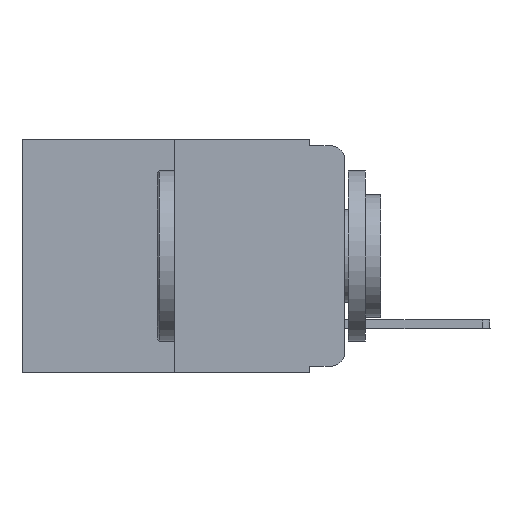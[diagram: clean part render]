
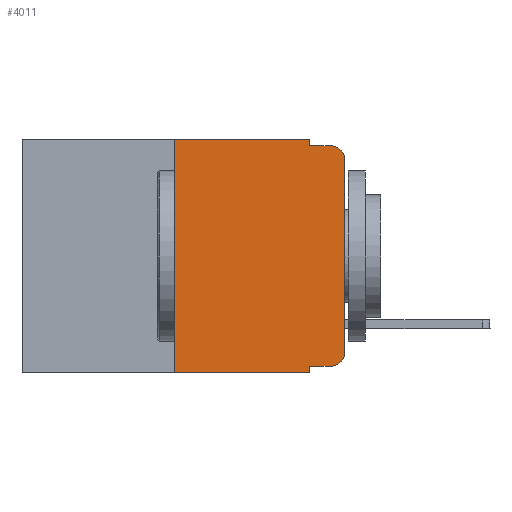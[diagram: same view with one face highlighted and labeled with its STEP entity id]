
A CAD part, left-side view. The second image highlights one B-rep face of the part: STEP entity #4011.
In plain terms, the highlighted planar face has unit normal (-1, 0, 0).
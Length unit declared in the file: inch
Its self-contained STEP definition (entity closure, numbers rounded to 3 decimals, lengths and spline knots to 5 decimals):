
#27 = VECTOR ( 'NONE', #8465, 39.37008 ) ;
#137 = CARTESIAN_POINT ( 'NONE',  ( 0., 0.25, 0. ) ) ;
#147 = DIRECTION ( 'NONE',  ( 0., -1., 0. ) ) ;
#211 = VECTOR ( 'NONE', #1115, 39.37008 ) ;
#227 = CARTESIAN_POINT ( 'NONE',  ( 0., 0.051, -0.01 ) ) ;
#622 = VERTEX_POINT ( 'NONE', #4128 ) ;
#785 = EDGE_CURVE ( 'NONE', #6028, #1741, #1272, .T. ) ;
#848 = VERTEX_POINT ( 'NONE', #7690 ) ;
#938 = CARTESIAN_POINT ( 'NONE',  ( 0., 0.473, 0. ) ) ;
#985 = CIRCLE ( 'NONE', #3263, 0.02 ) ;
#1009 = VECTOR ( 'NONE', #7620, 39.37008 ) ;
#1115 = DIRECTION ( 'NONE',  ( 0., 0., -1. ) ) ;
#1272 = LINE ( 'NONE', #227, #1009 ) ;
#1364 = CIRCLE ( 'NONE', #2346, 0.02 ) ;
#1446 = CARTESIAN_POINT ( 'NONE',  ( 0., 0.25, -0.343 ) ) ;
#1741 = VERTEX_POINT ( 'NONE', #6923 ) ;
#1876 = EDGE_CURVE ( 'NONE', #622, #10513, #1364, .T. ) ;
#1916 = CARTESIAN_POINT ( 'NONE',  ( 0., 0.473, 0. ) ) ;
#1956 = LINE ( 'NONE', #5800, #9907 ) ;
#2013 = LINE ( 'NONE', #9320, #211 ) ;
#2055 = VERTEX_POINT ( 'NONE', #137 ) ;
#2346 = AXIS2_PLACEMENT_3D ( 'NONE', #5459, #7097, #10304 ) ;
#2464 = CARTESIAN_POINT ( 'NONE',  ( 0., 0.02, -0.03 ) ) ;
#2688 = ORIENTED_EDGE ( 'NONE', *, *, #8754, .F. ) ;
#2755 = LINE ( 'NONE', #10289, #8506 ) ;
#2963 = DIRECTION ( 'NONE',  ( 0., 0., -1. ) ) ;
#3263 = AXIS2_PLACEMENT_3D ( 'NONE', #2464, #9793, #2963 ) ;
#3369 = CARTESIAN_POINT ( 'NONE',  ( 0., 0.051, 0. ) ) ;
#3418 = CARTESIAN_POINT ( 'NONE',  ( 0., 0., -0.03 ) ) ;
#3681 = DIRECTION ( 'NONE',  ( 0., 0., 1. ) ) ;
#3686 = EDGE_CURVE ( 'NONE', #10513, #10509, #2755, .T. ) ;
#4011 = ADVANCED_FACE ( 'NONE', ( #4802 ), #9938, .F. ) ;
#4128 = CARTESIAN_POINT ( 'NONE',  ( 0., 0.02, -0.333 ) ) ;
#4333 = ORIENTED_EDGE ( 'NONE', *, *, #5202, .T. ) ;
#4451 = VERTEX_POINT ( 'NONE', #1446 ) ;
#4654 = EDGE_CURVE ( 'NONE', #10509, #1741, #985, .T. ) ;
#4802 = FACE_OUTER_BOUND ( 'NONE', #8972, .T. ) ;
#5042 = EDGE_CURVE ( 'NONE', #6371, #848, #2013, .T. ) ;
#5116 = ORIENTED_EDGE ( 'NONE', *, *, #1876, .T. ) ;
#5119 = DIRECTION ( 'NONE',  ( 0., 0., -1. ) ) ;
#5202 = EDGE_CURVE ( 'NONE', #4451, #848, #7410, .T. ) ;
#5224 = VECTOR ( 'NONE', #7140, 39.37008 ) ;
#5459 = CARTESIAN_POINT ( 'NONE',  ( 0., 0.02, -0.313 ) ) ;
#5463 = CARTESIAN_POINT ( 'NONE',  ( 0., 0.473, -0.343 ) ) ;
#5565 = LINE ( 'NONE', #1916, #27 ) ;
#5712 = LINE ( 'NONE', #3369, #10300 ) ;
#5800 = CARTESIAN_POINT ( 'NONE',  ( 0., 0.051, -0.333 ) ) ;
#5867 = DIRECTION ( 'NONE',  ( 0., 0., -1. ) ) ;
#6028 = VERTEX_POINT ( 'NONE', #9392 ) ;
#6371 = VERTEX_POINT ( 'NONE', #9233 ) ;
#6533 = VERTEX_POINT ( 'NONE', #9372 ) ;
#6593 = ORIENTED_EDGE ( 'NONE', *, *, #4654, .T. ) ;
#6742 = ORIENTED_EDGE ( 'NONE', *, *, #8779, .F. ) ;
#6923 = CARTESIAN_POINT ( 'NONE',  ( 0., 0.02, -0.01 ) ) ;
#7097 = DIRECTION ( 'NONE',  ( -1., 0., 0. ) ) ;
#7140 = DIRECTION ( 'NONE',  ( 0., -1., 0. ) ) ;
#7410 = LINE ( 'NONE', #5463, #5224 ) ;
#7448 = CARTESIAN_POINT ( 'NONE',  ( 0., 0.25, 0. ) ) ;
#7620 = DIRECTION ( 'NONE',  ( 0., -1., 0. ) ) ;
#7690 = CARTESIAN_POINT ( 'NONE',  ( 0., 0.051, -0.343 ) ) ;
#7856 = AXIS2_PLACEMENT_3D ( 'NONE', #938, #9181, #5867 ) ;
#8150 = ORIENTED_EDGE ( 'NONE', *, *, #785, .F. ) ;
#8275 = ORIENTED_EDGE ( 'NONE', *, *, #5042, .F. ) ;
#8388 = VECTOR ( 'NONE', #3681, 39.37008 ) ;
#8465 = DIRECTION ( 'NONE',  ( 0., -1., 0. ) ) ;
#8506 = VECTOR ( 'NONE', #8693, 39.37008 ) ;
#8693 = DIRECTION ( 'NONE',  ( 0., 0., 1. ) ) ;
#8754 = EDGE_CURVE ( 'NONE', #6533, #6028, #5712, .T. ) ;
#8779 = EDGE_CURVE ( 'NONE', #4451, #2055, #9925, .T. ) ;
#8852 = ORIENTED_EDGE ( 'NONE', *, *, #3686, .T. ) ;
#8972 = EDGE_LOOP ( 'NONE', ( #8852, #6593, #8150, #2688, #9920, #6742, #4333, #8275, #9993, #5116 ) ) ;
#9181 = DIRECTION ( 'NONE',  ( 1., 0., 0. ) ) ;
#9233 = CARTESIAN_POINT ( 'NONE',  ( 0., 0.051, -0.333 ) ) ;
#9320 = CARTESIAN_POINT ( 'NONE',  ( 0., 0.051, 0. ) ) ;
#9372 = CARTESIAN_POINT ( 'NONE',  ( 0., 0.051, 0. ) ) ;
#9392 = CARTESIAN_POINT ( 'NONE',  ( 0., 0.051, -0.01 ) ) ;
#9793 = DIRECTION ( 'NONE',  ( -1., 0., 0. ) ) ;
#9907 = VECTOR ( 'NONE', #147, 39.37008 ) ;
#9920 = ORIENTED_EDGE ( 'NONE', *, *, #10043, .F. ) ;
#9925 = LINE ( 'NONE', #7448, #8388 ) ;
#9931 = EDGE_CURVE ( 'NONE', #6371, #622, #1956, .T. ) ;
#9938 = PLANE ( 'NONE',  #7856 ) ;
#9993 = ORIENTED_EDGE ( 'NONE', *, *, #9931, .T. ) ;
#9996 = CARTESIAN_POINT ( 'NONE',  ( 0., 0., -0.313 ) ) ;
#10043 = EDGE_CURVE ( 'NONE', #2055, #6533, #5565, .T. ) ;
#10289 = CARTESIAN_POINT ( 'NONE',  ( 0., 0., 0. ) ) ;
#10300 = VECTOR ( 'NONE', #5119, 39.37008 ) ;
#10304 = DIRECTION ( 'NONE',  ( 0., 0., -1. ) ) ;
#10509 = VERTEX_POINT ( 'NONE', #3418 ) ;
#10513 = VERTEX_POINT ( 'NONE', #9996 ) ;
